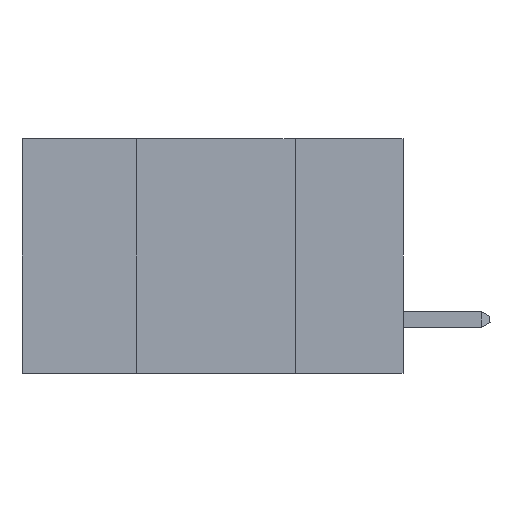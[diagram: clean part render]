
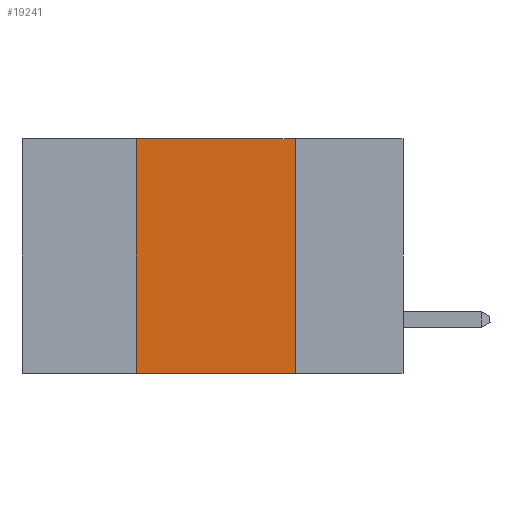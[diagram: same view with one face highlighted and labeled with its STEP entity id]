
A CAD part, left-side view. The second image highlights one B-rep face of the part: STEP entity #19241.
In plain terms, the highlighted planar face has unit normal (-1, 0, 0).
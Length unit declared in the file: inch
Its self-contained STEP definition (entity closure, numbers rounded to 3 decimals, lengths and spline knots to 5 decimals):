
#389 = LINE ( 'NONE', #1261, #18274 ) ;
#404 = EDGE_CURVE ( 'NONE', #16974, #17622, #12993, .T. ) ;
#1261 = CARTESIAN_POINT ( 'NONE',  ( 0., 0.42, 0. ) ) ;
#1598 = DIRECTION ( 'NONE',  ( 0., 0., 1. ) ) ;
#2451 = VERTEX_POINT ( 'NONE', #12393 ) ;
#3514 = VECTOR ( 'NONE', #6436, 39.37008 ) ;
#3683 = AXIS2_PLACEMENT_3D ( 'NONE', #8809, #13847, #17288 ) ;
#3863 = ORIENTED_EDGE ( 'NONE', *, *, #8658, .F. ) ;
#4422 = FACE_OUTER_BOUND ( 'NONE', #15834, .T. ) ;
#4852 = CARTESIAN_POINT ( 'NONE',  ( 0., 0.6, -0.37 ) ) ;
#5460 = LINE ( 'NONE', #14932, #8703 ) ;
#5602 = PLANE ( 'NONE',  #3683 ) ;
#5766 = EDGE_CURVE ( 'NONE', #16974, #12504, #389, .T. ) ;
#5778 = CARTESIAN_POINT ( 'NONE',  ( 0., 0.17, -0.37 ) ) ;
#6189 = VECTOR ( 'NONE', #12248, 39.37008 ) ;
#6436 = DIRECTION ( 'NONE',  ( 0., -1., 0. ) ) ;
#6865 = DIRECTION ( 'NONE',  ( 0., -1., 0. ) ) ;
#7944 = LINE ( 'NONE', #13806, #6189 ) ;
#8658 = EDGE_CURVE ( 'NONE', #12504, #2451, #5460, .T. ) ;
#8703 = VECTOR ( 'NONE', #6865, 39.37008 ) ;
#8809 = CARTESIAN_POINT ( 'NONE',  ( 0., 0.6, 0. ) ) ;
#8832 = EDGE_CURVE ( 'NONE', #2451, #17622, #7944, .T. ) ;
#12248 = DIRECTION ( 'NONE',  ( 0., 0., -1. ) ) ;
#12393 = CARTESIAN_POINT ( 'NONE',  ( 0., 0.17, 0. ) ) ;
#12504 = VERTEX_POINT ( 'NONE', #18319 ) ;
#12993 = LINE ( 'NONE', #4852, #3514 ) ;
#13806 = CARTESIAN_POINT ( 'NONE',  ( 0., 0.17, 0. ) ) ;
#13847 = DIRECTION ( 'NONE',  ( 1., 0., 0. ) ) ;
#14734 = ORIENTED_EDGE ( 'NONE', *, *, #404, .T. ) ;
#14922 = ORIENTED_EDGE ( 'NONE', *, *, #5766, .F. ) ;
#14932 = CARTESIAN_POINT ( 'NONE',  ( 0., 0.6, 0. ) ) ;
#15659 = ORIENTED_EDGE ( 'NONE', *, *, #8832, .F. ) ;
#15834 = EDGE_LOOP ( 'NONE', ( #15659, #3863, #14922, #14734 ) ) ;
#16974 = VERTEX_POINT ( 'NONE', #18523 ) ;
#17288 = DIRECTION ( 'NONE',  ( 0., 0., -1. ) ) ;
#17622 = VERTEX_POINT ( 'NONE', #5778 ) ;
#18274 = VECTOR ( 'NONE', #1598, 39.37008 ) ;
#18319 = CARTESIAN_POINT ( 'NONE',  ( 0., 0.42, 0. ) ) ;
#18523 = CARTESIAN_POINT ( 'NONE',  ( 0., 0.42, -0.37 ) ) ;
#19241 = ADVANCED_FACE ( 'NONE', ( #4422 ), #5602, .F. ) ;
